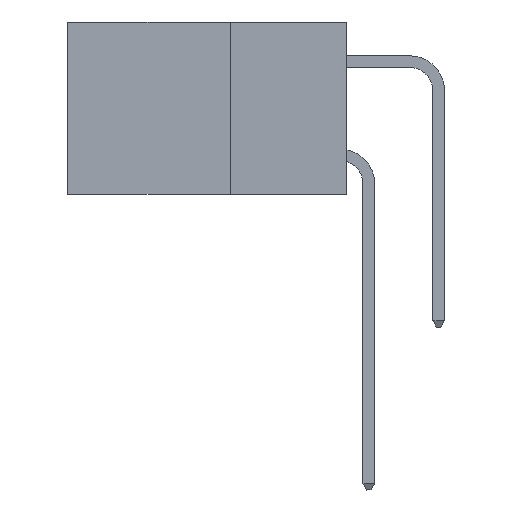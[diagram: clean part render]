
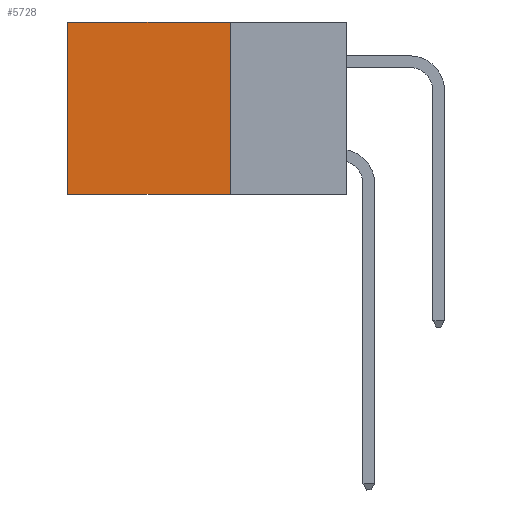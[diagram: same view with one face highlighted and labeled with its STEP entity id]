
A CAD part, left-side view. The second image highlights one B-rep face of the part: STEP entity #5728.
In plain terms, the highlighted planar face has unit normal (-1, 0, 0).
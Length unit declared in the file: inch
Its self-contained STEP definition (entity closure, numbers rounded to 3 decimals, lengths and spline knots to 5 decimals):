
#9 = EDGE_CURVE ( 'NONE', #19214, #17999, #14327, .T. ) ;
#120 = CARTESIAN_POINT ( 'NONE',  ( 0.2875, 0.25, 0. ) ) ;
#801 = CARTESIAN_POINT ( 'NONE',  ( 0.2875, 0.6, -0.37 ) ) ;
#1008 = LINE ( 'NONE', #10778, #18755 ) ;
#1801 = CARTESIAN_POINT ( 'NONE',  ( 0.2875, 0.6, 0. ) ) ;
#2210 = DIRECTION ( 'NONE',  ( 0., 1., 0. ) ) ;
#2495 = EDGE_CURVE ( 'NONE', #16049, #17999, #2944, .T. ) ;
#2944 = LINE ( 'NONE', #5016, #6508 ) ;
#3643 = CARTESIAN_POINT ( 'NONE',  ( 0.2875, 0.25, 0. ) ) ;
#3676 = VERTEX_POINT ( 'NONE', #16495 ) ;
#5016 = CARTESIAN_POINT ( 'NONE',  ( 0.2875, 0.6, 0. ) ) ;
#5424 = PLANE ( 'NONE',  #7463 ) ;
#5461 = ORIENTED_EDGE ( 'NONE', *, *, #5852, .F. ) ;
#5728 = ADVANCED_FACE ( 'NONE', ( #21350 ), #5424, .F. ) ;
#5852 = EDGE_CURVE ( 'NONE', #3676, #19214, #1008, .T. ) ;
#6508 = VECTOR ( 'NONE', #22023, 39.37008 ) ;
#7158 = DIRECTION ( 'NONE',  ( 0., 0., -1. ) ) ;
#7463 = AXIS2_PLACEMENT_3D ( 'NONE', #3643, #17316, #7158 ) ;
#9156 = DIRECTION ( 'NONE',  ( 0., 0., -1. ) ) ;
#9803 = VECTOR ( 'NONE', #2210, 39.37008 ) ;
#10778 = CARTESIAN_POINT ( 'NONE',  ( 0.2875, 0.25, 0. ) ) ;
#11046 = EDGE_CURVE ( 'NONE', #3676, #16049, #18712, .T. ) ;
#11121 = ORIENTED_EDGE ( 'NONE', *, *, #2495, .T. ) ;
#12221 = DIRECTION ( 'NONE',  ( 0., 1., 0. ) ) ;
#14217 = VECTOR ( 'NONE', #12221, 39.37008 ) ;
#14327 = LINE ( 'NONE', #21129, #9803 ) ;
#14336 = ORIENTED_EDGE ( 'NONE', *, *, #9, .F. ) ;
#14818 = CARTESIAN_POINT ( 'NONE',  ( 0.2875, 0.25, -0.37 ) ) ;
#16049 = VERTEX_POINT ( 'NONE', #1801 ) ;
#16495 = CARTESIAN_POINT ( 'NONE',  ( 0.2875, 0.25, 0. ) ) ;
#17207 = EDGE_LOOP ( 'NONE', ( #11121, #14336, #5461, #20213 ) ) ;
#17316 = DIRECTION ( 'NONE',  ( 1., 0., 0. ) ) ;
#17999 = VERTEX_POINT ( 'NONE', #801 ) ;
#18712 = LINE ( 'NONE', #120, #14217 ) ;
#18755 = VECTOR ( 'NONE', #9156, 39.37008 ) ;
#19214 = VERTEX_POINT ( 'NONE', #14818 ) ;
#20213 = ORIENTED_EDGE ( 'NONE', *, *, #11046, .T. ) ;
#21129 = CARTESIAN_POINT ( 'NONE',  ( 0.2875, 0.25, -0.37 ) ) ;
#21350 = FACE_OUTER_BOUND ( 'NONE', #17207, .T. ) ;
#22023 = DIRECTION ( 'NONE',  ( 0., 0., -1. ) ) ;
